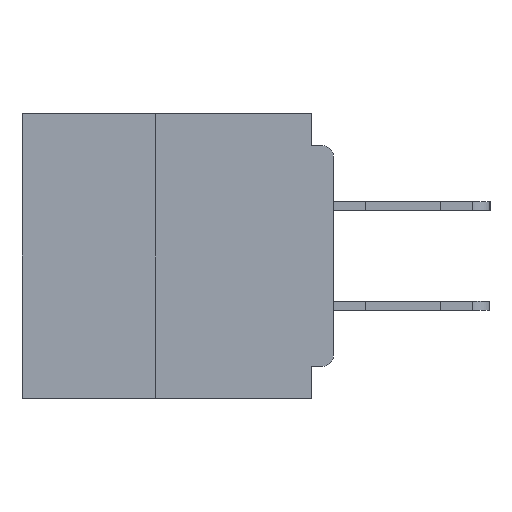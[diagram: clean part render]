
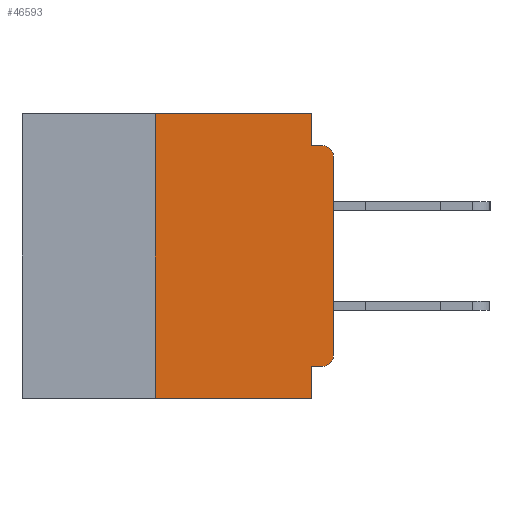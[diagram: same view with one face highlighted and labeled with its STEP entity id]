
A CAD part, left-side view. The second image highlights one B-rep face of the part: STEP entity #46593.
In plain terms, the highlighted planar face has unit normal (-1, 0, 0).
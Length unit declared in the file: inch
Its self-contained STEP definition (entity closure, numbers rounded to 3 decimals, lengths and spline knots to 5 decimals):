
#688 = EDGE_CURVE ( 'NONE', #16059, #16479, #29780, .T. ) ;
#768 = VECTOR ( 'NONE', #42190, 39.37008 ) ;
#1036 = ORIENTED_EDGE ( 'NONE', *, *, #42947, .F. ) ;
#1208 = EDGE_CURVE ( 'NONE', #52267, #27937, #34481, .T. ) ;
#3536 = EDGE_CURVE ( 'NONE', #24150, #6981, #24049, .T. ) ;
#5848 = ORIENTED_EDGE ( 'NONE', *, *, #3536, .T. ) ;
#6365 = VECTOR ( 'NONE', #16556, 39.37008 ) ;
#6493 = DIRECTION ( 'NONE',  ( 1., 0., 0. ) ) ;
#6670 = DIRECTION ( 'NONE',  ( 0., 0., 1. ) ) ;
#6896 = CARTESIAN_POINT ( 'NONE',  ( 0., 0.031, -0.045 ) ) ;
#6981 = VERTEX_POINT ( 'NONE', #30568 ) ;
#8146 = VERTEX_POINT ( 'NONE', #6896 ) ;
#8401 = EDGE_LOOP ( 'NONE', ( #16780, #32496, #1036, #22683, #42466, #22955, #5848, #30522, #36610, #44182 ) ) ;
#8491 = CARTESIAN_POINT ( 'NONE',  ( 0., 0.437, 0. ) ) ;
#13078 = AXIS2_PLACEMENT_3D ( 'NONE', #32674, #6493, #37063 ) ;
#13153 = DIRECTION ( 'NONE',  ( 0., -1., 0. ) ) ;
#14776 = CARTESIAN_POINT ( 'NONE',  ( 0., 0.25, -0.4 ) ) ;
#15295 = CARTESIAN_POINT ( 'NONE',  ( 0., 0.25, -0.4 ) ) ;
#16059 = VERTEX_POINT ( 'NONE', #36556 ) ;
#16479 = VERTEX_POINT ( 'NONE', #49002 ) ;
#16556 = DIRECTION ( 'NONE',  ( 0., 0., 1. ) ) ;
#16780 = ORIENTED_EDGE ( 'NONE', *, *, #54843, .T. ) ;
#19584 = DIRECTION ( 'NONE',  ( -1., 0., 0. ) ) ;
#20042 = VECTOR ( 'NONE', #50066, 39.37008 ) ;
#20293 = DIRECTION ( 'NONE',  ( 0., -1., 0. ) ) ;
#20929 = VECTOR ( 'NONE', #13153, 39.37008 ) ;
#22683 = ORIENTED_EDGE ( 'NONE', *, *, #56309, .F. ) ;
#22955 = ORIENTED_EDGE ( 'NONE', *, *, #44579, .F. ) ;
#24024 = LINE ( 'NONE', #53126, #44484 ) ;
#24049 = LINE ( 'NONE', #41976, #768 ) ;
#24150 = VERTEX_POINT ( 'NONE', #14776 ) ;
#26812 = CARTESIAN_POINT ( 'NONE',  ( 0., 0.031, -0.4 ) ) ;
#27344 = VERTEX_POINT ( 'NONE', #42325 ) ;
#27937 = VERTEX_POINT ( 'NONE', #41873 ) ;
#28644 = VERTEX_POINT ( 'NONE', #34241 ) ;
#29173 = FACE_OUTER_BOUND ( 'NONE', #8401, .T. ) ;
#29544 = CARTESIAN_POINT ( 'NONE',  ( 0., 0., 0. ) ) ;
#29780 = LINE ( 'NONE', #8491, #51696 ) ;
#30522 = ORIENTED_EDGE ( 'NONE', *, *, #36862, .F. ) ;
#30568 = CARTESIAN_POINT ( 'NONE',  ( 0., 0.031, -0.4 ) ) ;
#30864 = CIRCLE ( 'NONE', #49121, 0.015 ) ;
#32475 = LINE ( 'NONE', #52371, #20929 ) ;
#32496 = ORIENTED_EDGE ( 'NONE', *, *, #39255, .T. ) ;
#32674 = CARTESIAN_POINT ( 'NONE',  ( 0., 0.437, 0. ) ) ;
#33782 = AXIS2_PLACEMENT_3D ( 'NONE', #43473, #43345, #43340 ) ;
#34241 = CARTESIAN_POINT ( 'NONE',  ( 0., 0.015, -0.045 ) ) ;
#34481 = CIRCLE ( 'NONE', #33782, 0.015 ) ;
#34510 = LINE ( 'NONE', #26812, #46151 ) ;
#36556 = CARTESIAN_POINT ( 'NONE',  ( 0., 0.25, 0. ) ) ;
#36610 = ORIENTED_EDGE ( 'NONE', *, *, #38177, .F. ) ;
#36862 = EDGE_CURVE ( 'NONE', #52002, #6981, #34510, .T. ) ;
#37063 = DIRECTION ( 'NONE',  ( 0., 0., -1. ) ) ;
#38177 = EDGE_CURVE ( 'NONE', #52267, #52002, #54911, .T. ) ;
#39255 = EDGE_CURVE ( 'NONE', #27344, #28644, #30864, .T. ) ;
#41213 = CARTESIAN_POINT ( 'NONE',  ( 0., 0., -0.355 ) ) ;
#41220 = LINE ( 'NONE', #29544, #6365 ) ;
#41246 = VECTOR ( 'NONE', #6670, 39.37008 ) ;
#41873 = CARTESIAN_POINT ( 'NONE',  ( 0., 0., -0.34 ) ) ;
#41976 = CARTESIAN_POINT ( 'NONE',  ( 0., 0.437, -0.4 ) ) ;
#42190 = DIRECTION ( 'NONE',  ( 0., -1., 0. ) ) ;
#42325 = CARTESIAN_POINT ( 'NONE',  ( 0., 0., -0.06 ) ) ;
#42466 = ORIENTED_EDGE ( 'NONE', *, *, #688, .F. ) ;
#42947 = EDGE_CURVE ( 'NONE', #8146, #28644, #32475, .T. ) ;
#43340 = DIRECTION ( 'NONE',  ( 0., 0., -1. ) ) ;
#43345 = DIRECTION ( 'NONE',  ( -1., 0., 0. ) ) ;
#43473 = CARTESIAN_POINT ( 'NONE',  ( 0., 0.015, -0.34 ) ) ;
#43558 = CARTESIAN_POINT ( 'NONE',  ( 0., 0.015, -0.355 ) ) ;
#44182 = ORIENTED_EDGE ( 'NONE', *, *, #1208, .T. ) ;
#44484 = VECTOR ( 'NONE', #44488, 39.37008 ) ;
#44488 = DIRECTION ( 'NONE',  ( 0., 0., -1. ) ) ;
#44579 = EDGE_CURVE ( 'NONE', #24150, #16059, #52936, .T. ) ;
#45712 = CARTESIAN_POINT ( 'NONE',  ( 0., 0.015, -0.06 ) ) ;
#46151 = VECTOR ( 'NONE', #48606, 39.37008 ) ;
#46593 = ADVANCED_FACE ( 'NONE', ( #29173 ), #50107, .F. ) ;
#48606 = DIRECTION ( 'NONE',  ( 0., 0., -1. ) ) ;
#49002 = CARTESIAN_POINT ( 'NONE',  ( 0., 0.031, 0. ) ) ;
#49121 = AXIS2_PLACEMENT_3D ( 'NONE', #45712, #19584, #50152 ) ;
#50066 = DIRECTION ( 'NONE',  ( 0., 1., 0. ) ) ;
#50107 = PLANE ( 'NONE',  #13078 ) ;
#50152 = DIRECTION ( 'NONE',  ( 0., 0., -1. ) ) ;
#50514 = CARTESIAN_POINT ( 'NONE',  ( 0., 0.031, -0.355 ) ) ;
#51696 = VECTOR ( 'NONE', #20293, 39.37008 ) ;
#52002 = VERTEX_POINT ( 'NONE', #50514 ) ;
#52267 = VERTEX_POINT ( 'NONE', #43558 ) ;
#52371 = CARTESIAN_POINT ( 'NONE',  ( 0., 0., -0.045 ) ) ;
#52936 = LINE ( 'NONE', #15295, #41246 ) ;
#53126 = CARTESIAN_POINT ( 'NONE',  ( 0., 0.031, 0. ) ) ;
#54843 = EDGE_CURVE ( 'NONE', #27937, #27344, #41220, .T. ) ;
#54911 = LINE ( 'NONE', #41213, #20042 ) ;
#56309 = EDGE_CURVE ( 'NONE', #16479, #8146, #24024, .T. ) ;
